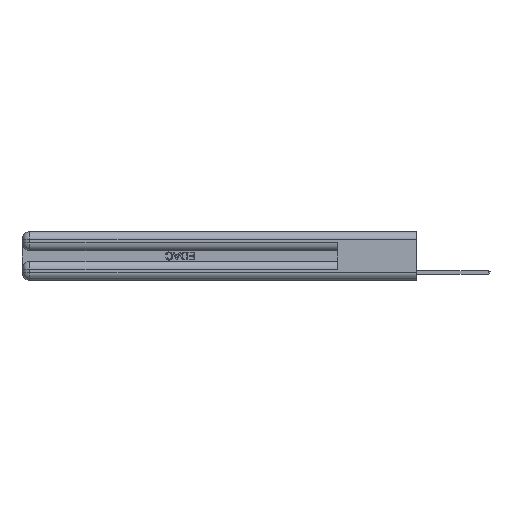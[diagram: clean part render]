
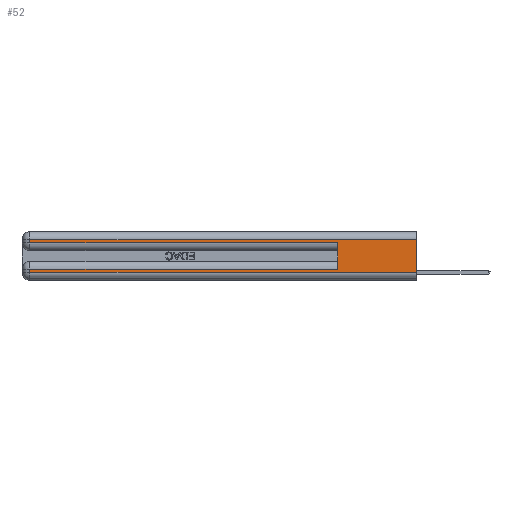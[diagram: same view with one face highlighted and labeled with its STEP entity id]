
A CAD part, left-side view. The second image highlights one B-rep face of the part: STEP entity #52.
In plain terms, the highlighted planar face has unit normal (-1, 0, 0).
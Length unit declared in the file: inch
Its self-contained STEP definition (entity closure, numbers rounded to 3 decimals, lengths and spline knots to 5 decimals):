
#52 = ADVANCED_FACE ( 'NONE', ( #20047 ), #20676, .F. ) ;
#367 = CARTESIAN_POINT ( 'NONE',  ( 0., 0., 0.06 ) ) ;
#774 = CARTESIAN_POINT ( 'NONE',  ( 0., 0., 0.31 ) ) ;
#1212 = VECTOR ( 'NONE', #20762, 39.37008 ) ;
#2457 = CARTESIAN_POINT ( 'NONE',  ( 0., 2.94, 0.285 ) ) ;
#2892 = ORIENTED_EDGE ( 'NONE', *, *, #6021, .F. ) ;
#2959 = EDGE_LOOP ( 'NONE', ( #5267, #27519, #25035, #13588, #2892, #10882, #27865, #6337 ) ) ;
#3149 = EDGE_CURVE ( 'NONE', #21772, #22427, #29984, .T. ) ;
#3200 = EDGE_CURVE ( 'NONE', #21772, #17910, #14034, .T. ) ;
#4490 = LINE ( 'NONE', #367, #24738 ) ;
#4527 = VECTOR ( 'NONE', #25634, 39.37008 ) ;
#5138 = LINE ( 'NONE', #26567, #14826 ) ;
#5267 = ORIENTED_EDGE ( 'NONE', *, *, #3149, .F. ) ;
#6021 = EDGE_CURVE ( 'NONE', #26423, #11752, #29028, .T. ) ;
#6337 = ORIENTED_EDGE ( 'NONE', *, *, #10456, .T. ) ;
#6978 = DIRECTION ( 'NONE',  ( 0., 0., -1. ) ) ;
#7278 = EDGE_CURVE ( 'NONE', #17910, #21025, #10548, .T. ) ;
#8063 = DIRECTION ( 'NONE',  ( 0., 0., -1. ) ) ;
#8805 = CARTESIAN_POINT ( 'NONE',  ( 0., 0., 0.285 ) ) ;
#9232 = LINE ( 'NONE', #21510, #4527 ) ;
#10255 = VERTEX_POINT ( 'NONE', #24453 ) ;
#10456 = EDGE_CURVE ( 'NONE', #23296, #22427, #4490, .T. ) ;
#10548 = LINE ( 'NONE', #18210, #1212 ) ;
#10882 = ORIENTED_EDGE ( 'NONE', *, *, #15494, .T. ) ;
#10945 = VECTOR ( 'NONE', #20917, 39.37008 ) ;
#11656 = AXIS2_PLACEMENT_3D ( 'NONE', #23038, #25222, #8063 ) ;
#11752 = VERTEX_POINT ( 'NONE', #13045 ) ;
#12015 = CARTESIAN_POINT ( 'NONE',  ( 0., 0.6, 0.085 ) ) ;
#13045 = CARTESIAN_POINT ( 'NONE',  ( 0., 0.6, 0.285 ) ) ;
#13403 = CARTESIAN_POINT ( 'NONE',  ( 0., 0., 0.37 ) ) ;
#13588 = ORIENTED_EDGE ( 'NONE', *, *, #30929, .T. ) ;
#14034 = LINE ( 'NONE', #774, #19486 ) ;
#14826 = VECTOR ( 'NONE', #6978, 39.37008 ) ;
#15494 = EDGE_CURVE ( 'NONE', #26423, #10255, #9232, .T. ) ;
#15779 = VECTOR ( 'NONE', #29736, 39.37008 ) ;
#17824 = CARTESIAN_POINT ( 'NONE',  ( 0., 2.94, 0.06 ) ) ;
#17910 = VERTEX_POINT ( 'NONE', #27577 ) ;
#18210 = CARTESIAN_POINT ( 'NONE',  ( 0., 2.94, 0.37 ) ) ;
#19486 = VECTOR ( 'NONE', #25584, 39.37008 ) ;
#19577 = LINE ( 'NONE', #8805, #27356 ) ;
#19870 = CARTESIAN_POINT ( 'NONE',  ( 0., 0.6, 0.145 ) ) ;
#20047 = FACE_OUTER_BOUND ( 'NONE', #2959, .T. ) ;
#20676 = PLANE ( 'NONE',  #11656 ) ;
#20762 = DIRECTION ( 'NONE',  ( 0., 0., -1. ) ) ;
#20917 = DIRECTION ( 'NONE',  ( 0., 0., -1. ) ) ;
#21025 = VERTEX_POINT ( 'NONE', #2457 ) ;
#21510 = CARTESIAN_POINT ( 'NONE',  ( 0., 0., 0.085 ) ) ;
#21772 = VERTEX_POINT ( 'NONE', #27750 ) ;
#22427 = VERTEX_POINT ( 'NONE', #29511 ) ;
#23038 = CARTESIAN_POINT ( 'NONE',  ( 0., 0., 0.37 ) ) ;
#23296 = VERTEX_POINT ( 'NONE', #17824 ) ;
#24117 = DIRECTION ( 'NONE',  ( 0., -1., 0. ) ) ;
#24453 = CARTESIAN_POINT ( 'NONE',  ( 0., 2.94, 0.085 ) ) ;
#24738 = VECTOR ( 'NONE', #30710, 39.37008 ) ;
#25035 = ORIENTED_EDGE ( 'NONE', *, *, #7278, .T. ) ;
#25222 = DIRECTION ( 'NONE',  ( 1., 0., 0. ) ) ;
#25584 = DIRECTION ( 'NONE',  ( 0., 1., 0. ) ) ;
#25634 = DIRECTION ( 'NONE',  ( 0., 1., 0. ) ) ;
#26423 = VERTEX_POINT ( 'NONE', #12015 ) ;
#26567 = CARTESIAN_POINT ( 'NONE',  ( 0., 2.94, 0.37 ) ) ;
#27356 = VECTOR ( 'NONE', #24117, 39.37008 ) ;
#27519 = ORIENTED_EDGE ( 'NONE', *, *, #3200, .T. ) ;
#27577 = CARTESIAN_POINT ( 'NONE',  ( 0., 2.94, 0.31 ) ) ;
#27750 = CARTESIAN_POINT ( 'NONE',  ( 0., 0., 0.31 ) ) ;
#27865 = ORIENTED_EDGE ( 'NONE', *, *, #31686, .T. ) ;
#29028 = LINE ( 'NONE', #19870, #15779 ) ;
#29511 = CARTESIAN_POINT ( 'NONE',  ( 0., 0., 0.06 ) ) ;
#29736 = DIRECTION ( 'NONE',  ( 0., 0., 1. ) ) ;
#29984 = LINE ( 'NONE', #13403, #10945 ) ;
#30710 = DIRECTION ( 'NONE',  ( 0., -1., 0. ) ) ;
#30929 = EDGE_CURVE ( 'NONE', #21025, #11752, #19577, .T. ) ;
#31686 = EDGE_CURVE ( 'NONE', #10255, #23296, #5138, .T. ) ;
